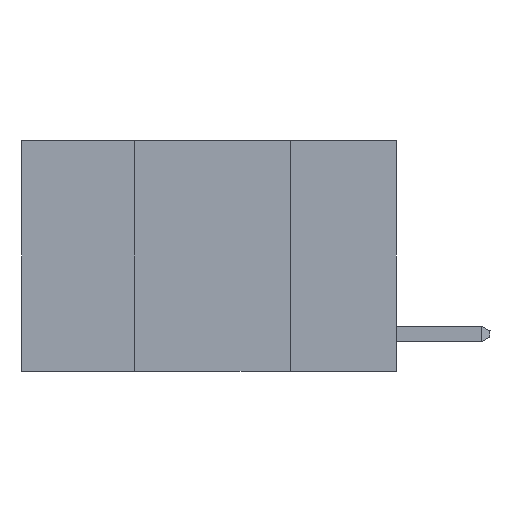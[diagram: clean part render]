
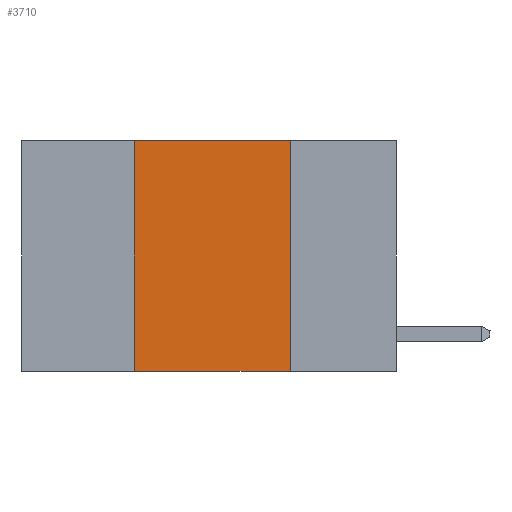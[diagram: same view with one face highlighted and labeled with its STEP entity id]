
A CAD part, left-side view. The second image highlights one B-rep face of the part: STEP entity #3710.
In plain terms, the highlighted planar face has unit normal (-1, 0, 0).
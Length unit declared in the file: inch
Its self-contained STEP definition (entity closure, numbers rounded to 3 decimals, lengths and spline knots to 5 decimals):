
#153 = AXIS2_PLACEMENT_3D ( 'NONE', #410, #529, #11934 ) ;
#284 = LINE ( 'NONE', #2500, #8002 ) ;
#407 = ORIENTED_EDGE ( 'NONE', *, *, #4083, .T. ) ;
#410 = CARTESIAN_POINT ( 'NONE',  ( 0., 0.6, 0. ) ) ;
#458 = ORIENTED_EDGE ( 'NONE', *, *, #2073, .F. ) ;
#529 = DIRECTION ( 'NONE',  ( 1., 0., 0. ) ) ;
#1086 = DIRECTION ( 'NONE',  ( 0., -1., 0. ) ) ;
#1249 = VECTOR ( 'NONE', #1086, 39.37008 ) ;
#1488 = DIRECTION ( 'NONE',  ( 0., -1., 0. ) ) ;
#2073 = EDGE_CURVE ( 'NONE', #4564, #7289, #11237, .T. ) ;
#2427 = PLANE ( 'NONE',  #153 ) ;
#2500 = CARTESIAN_POINT ( 'NONE',  ( 0., 0.42, 0. ) ) ;
#2731 = ORIENTED_EDGE ( 'NONE', *, *, #6552, .F. ) ;
#3695 = VECTOR ( 'NONE', #1488, 39.37008 ) ;
#3710 = ADVANCED_FACE ( 'NONE', ( #7927 ), #2427, .F. ) ;
#4083 = EDGE_CURVE ( 'NONE', #4486, #5014, #5903, .T. ) ;
#4486 = VERTEX_POINT ( 'NONE', #7153 ) ;
#4544 = CARTESIAN_POINT ( 'NONE',  ( 0., 0.17, 0. ) ) ;
#4564 = VERTEX_POINT ( 'NONE', #8994 ) ;
#5014 = VERTEX_POINT ( 'NONE', #7207 ) ;
#5425 = LINE ( 'NONE', #10662, #10592 ) ;
#5616 = EDGE_LOOP ( 'NONE', ( #9067, #458, #2731, #407 ) ) ;
#5903 = LINE ( 'NONE', #6644, #1249 ) ;
#5965 = DIRECTION ( 'NONE',  ( 0., 0., -1. ) ) ;
#6552 = EDGE_CURVE ( 'NONE', #4486, #4564, #284, .T. ) ;
#6644 = CARTESIAN_POINT ( 'NONE',  ( 0., 0.6, -0.37 ) ) ;
#7153 = CARTESIAN_POINT ( 'NONE',  ( 0., 0.42, -0.37 ) ) ;
#7207 = CARTESIAN_POINT ( 'NONE',  ( 0., 0.17, -0.37 ) ) ;
#7289 = VERTEX_POINT ( 'NONE', #4544 ) ;
#7927 = FACE_OUTER_BOUND ( 'NONE', #5616, .T. ) ;
#8002 = VECTOR ( 'NONE', #12129, 39.37008 ) ;
#8994 = CARTESIAN_POINT ( 'NONE',  ( 0., 0.42, 0. ) ) ;
#9067 = ORIENTED_EDGE ( 'NONE', *, *, #11153, .F. ) ;
#10592 = VECTOR ( 'NONE', #5965, 39.37008 ) ;
#10662 = CARTESIAN_POINT ( 'NONE',  ( 0., 0.17, 0. ) ) ;
#11153 = EDGE_CURVE ( 'NONE', #7289, #5014, #5425, .T. ) ;
#11237 = LINE ( 'NONE', #11862, #3695 ) ;
#11862 = CARTESIAN_POINT ( 'NONE',  ( 0., 0.6, 0. ) ) ;
#11934 = DIRECTION ( 'NONE',  ( 0., 0., -1. ) ) ;
#12129 = DIRECTION ( 'NONE',  ( 0., 0., 1. ) ) ;
